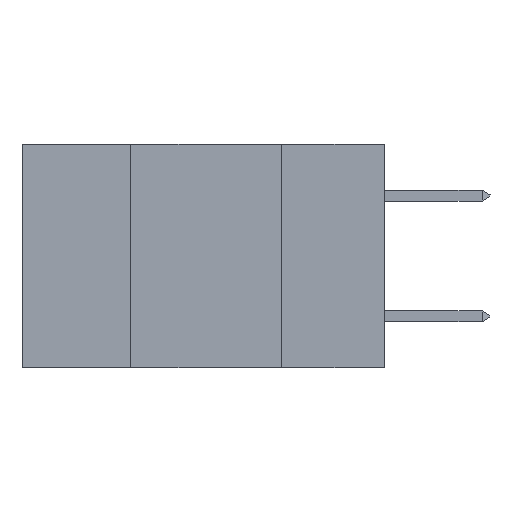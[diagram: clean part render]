
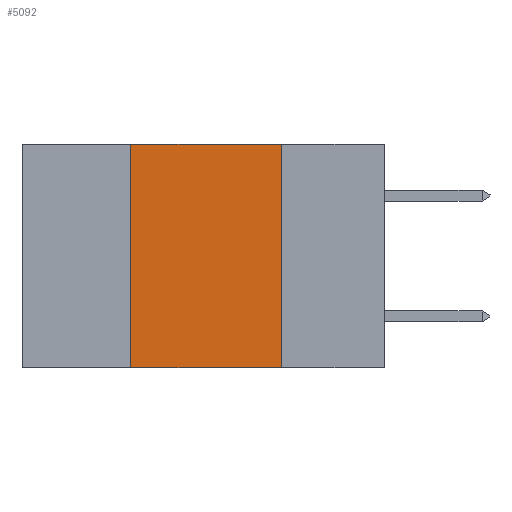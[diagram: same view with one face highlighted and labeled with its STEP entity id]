
A CAD part, left-side view. The second image highlights one B-rep face of the part: STEP entity #5092.
In plain terms, the highlighted planar face has unit normal (-1, 0, 0).
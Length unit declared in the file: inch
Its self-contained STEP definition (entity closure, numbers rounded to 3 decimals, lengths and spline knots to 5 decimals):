
#1479 = VECTOR ( 'NONE', #20055, 39.37008 ) ;
#2417 = EDGE_LOOP ( 'NONE', ( #12902, #25439, #8842, #22740 ) ) ;
#3382 = DIRECTION ( 'NONE',  ( 0., -1., 0. ) ) ;
#4188 = VECTOR ( 'NONE', #7769, 39.37008 ) ;
#4192 = VECTOR ( 'NONE', #5631, 39.37008 ) ;
#5092 = ADVANCED_FACE ( 'NONE', ( #19758 ), #16532, .F. ) ;
#5442 = EDGE_CURVE ( 'NONE', #25083, #10050, #16763, .T. ) ;
#5631 = DIRECTION ( 'NONE',  ( 0., 0., -1. ) ) ;
#6868 = CARTESIAN_POINT ( 'NONE',  ( 0., 0.42, 0. ) ) ;
#7769 = DIRECTION ( 'NONE',  ( 0., -1., 0. ) ) ;
#8842 = ORIENTED_EDGE ( 'NONE', *, *, #5442, .F. ) ;
#9541 = CARTESIAN_POINT ( 'NONE',  ( 0., 0.6, 0. ) ) ;
#10050 = VERTEX_POINT ( 'NONE', #6868 ) ;
#11726 = VECTOR ( 'NONE', #3382, 39.37008 ) ;
#12902 = ORIENTED_EDGE ( 'NONE', *, *, #22448, .F. ) ;
#14061 = CARTESIAN_POINT ( 'NONE',  ( 0., 0.6, -0.37 ) ) ;
#14477 = CARTESIAN_POINT ( 'NONE',  ( 0., 0.17, 0. ) ) ;
#14985 = CARTESIAN_POINT ( 'NONE',  ( 0., 0.17, -0.37 ) ) ;
#15705 = CARTESIAN_POINT ( 'NONE',  ( 0., 0.42, -0.37 ) ) ;
#16278 = EDGE_CURVE ( 'NONE', #25083, #18656, #17811, .T. ) ;
#16446 = DIRECTION ( 'NONE',  ( 1., 0., 0. ) ) ;
#16532 = PLANE ( 'NONE',  #26254 ) ;
#16763 = LINE ( 'NONE', #26305, #1479 ) ;
#17033 = VERTEX_POINT ( 'NONE', #22994 ) ;
#17811 = LINE ( 'NONE', #14061, #4188 ) ;
#18489 = EDGE_CURVE ( 'NONE', #10050, #17033, #20992, .T. ) ;
#18656 = VERTEX_POINT ( 'NONE', #14985 ) ;
#19758 = FACE_OUTER_BOUND ( 'NONE', #2417, .T. ) ;
#20055 = DIRECTION ( 'NONE',  ( 0., 0., 1. ) ) ;
#20698 = DIRECTION ( 'NONE',  ( 0., 0., -1. ) ) ;
#20992 = LINE ( 'NONE', #9541, #11726 ) ;
#22448 = EDGE_CURVE ( 'NONE', #17033, #18656, #27103, .T. ) ;
#22740 = ORIENTED_EDGE ( 'NONE', *, *, #16278, .T. ) ;
#22910 = CARTESIAN_POINT ( 'NONE',  ( 0., 0.6, 0. ) ) ;
#22994 = CARTESIAN_POINT ( 'NONE',  ( 0., 0.17, 0. ) ) ;
#25083 = VERTEX_POINT ( 'NONE', #15705 ) ;
#25439 = ORIENTED_EDGE ( 'NONE', *, *, #18489, .F. ) ;
#26254 = AXIS2_PLACEMENT_3D ( 'NONE', #22910, #16446, #20698 ) ;
#26305 = CARTESIAN_POINT ( 'NONE',  ( 0., 0.42, 0. ) ) ;
#27103 = LINE ( 'NONE', #14477, #4192 ) ;
